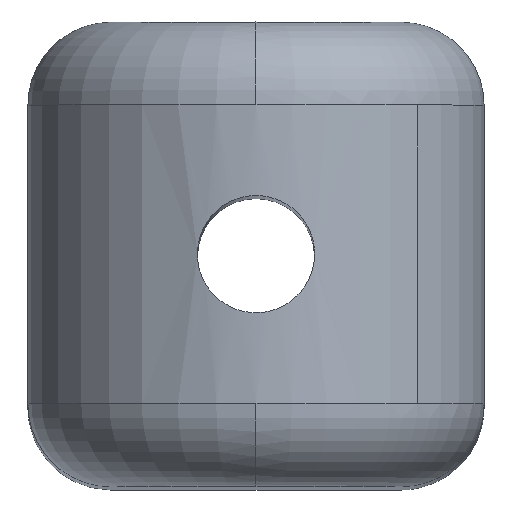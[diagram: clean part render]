
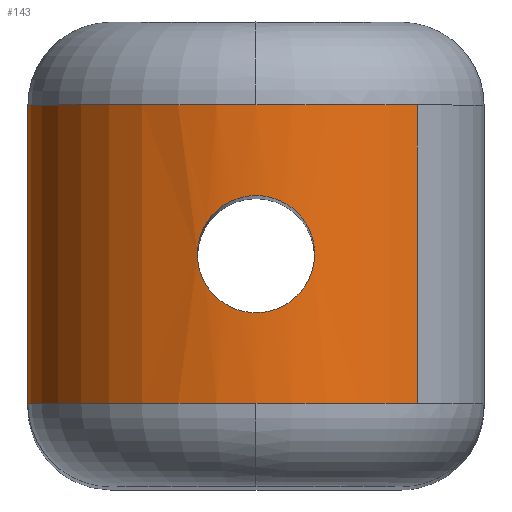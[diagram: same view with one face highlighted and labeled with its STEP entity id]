
A CAD part, top view. The second image highlights one B-rep face of the part: STEP entity #143.
In plain terms, the highlighted cylindrical face has radius 11 mm (diameter 22 mm), a partial arc.
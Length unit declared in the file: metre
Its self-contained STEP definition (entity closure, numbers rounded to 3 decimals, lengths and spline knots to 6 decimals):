
#143=ADVANCED_FACE('0:40',(#271,#272),#273,.T.);
#271=FACE_OUTER_BOUND('',#383,.T.);
#272=FACE_BOUND('',#384,.T.);
#273=CYLINDRICAL_SURFACE('',#385,0.011);
#383=EDGE_LOOP('',(#640,#641,#642,#643,#644,#645));
#384=EDGE_LOOP('',(#646,#647));
#385=AXIS2_PLACEMENT_3D('',#648,#649,#650);
#640=ORIENTED_EDGE('',*,*,#654,.T.);
#641=ORIENTED_EDGE('',*,*,#660,.F.);
#642=ORIENTED_EDGE('',*,*,#751,.F.);
#643=ORIENTED_EDGE('',*,*,#749,.F.);
#644=ORIENTED_EDGE('',*,*,#747,.F.);
#645=ORIENTED_EDGE('',*,*,#669,.F.);
#646=ORIENTED_EDGE('',*,*,#716,.T.);
#647=ORIENTED_EDGE('',*,*,#702,.T.);
#648=CARTESIAN_POINT('',(0.,0.0,0.099));
#649=DIRECTION('',(0.0,-1.0,0.0));
#650=DIRECTION('',(0.707,0.0,0.707));
#654=EDGE_CURVE('',#755,#756,#757,.T.);
#660=EDGE_CURVE('0:184',#764,#756,#767,.T.);
#669=EDGE_CURVE('0:199',#755,#775,#782,.T.);
#702=EDGE_CURVE('0:4471',#834,#831,#835,.T.);
#716=EDGE_CURVE('0:4471',#831,#834,#854,.T.);
#747=EDGE_CURVE('0:199',#775,#873,#890,.T.);
#749=EDGE_CURVE('0:328',#873,#880,#892,.T.);
#751=EDGE_CURVE('0:184',#880,#764,#894,.T.);
#755=VERTEX_POINT('',#898);
#756=VERTEX_POINT('',#899);
#757=LINE('',#900,#901);
#764=VERTEX_POINT('',#909);
#767=CIRCLE('',#912,0.011);
#775=VERTEX_POINT('',#920);
#782=CIRCLE('',#927,0.011);
#831=VERTEX_POINT('',#990);
#834=VERTEX_POINT('',#994);
#835=B_SPLINE_CURVE_WITH_KNOTS('',3,(#995,#996,#997,#998,#999,#1000,#1001,#1002,#1003,#1004,#1005,#1006,#1007,#1008,#1009,#1010,#1011,#1012,#1013,#1014,#1015,#1016,#1017,#1018,#1019,#1020,#1021,#1022,#1023,#1024,#1025,#1026,#1027,#1028),.UNSPECIFIED.,.F.,.F.,(4,3,3,3,3,3,3,3,3,3,3,4),(0.008555,0.009653,0.010546,0.011007,0.0121,0.012752,0.013258,0.014269,0.014853,0.015323,0.016413,0.017109),.UNSPECIFIED.);
#854=B_SPLINE_CURVE_WITH_KNOTS('',3,(#1050,#1051,#1052,#1053,#1054,#1055,#1056,#1057,#1058,#1059,#1060,#1061,#1062,#1063,#1064,#1065,#1066,#1067,#1068,#1069,#1070,#1071,#1072,#1073,#1074,#1075,#1076,#1077,#1078,#1079,#1080,#1081,#1082,#1083),.UNSPECIFIED.,.F.,.F.,(4,3,3,3,3,3,3,3,3,3,3,4),(0.0,0.001098,0.001991,0.002452,0.003546,0.004197,0.004703,0.005714,0.006298,0.006768,0.007859,0.008555),.UNSPECIFIED.);
#873=VERTEX_POINT('',#1105);
#880=VERTEX_POINT('',#1115);
#890=CIRCLE('',#1127,0.011);
#892=LINE('',#1129,#1130);
#894=CIRCLE('',#1132,0.011);
#898=CARTESIAN_POINT('',(0.007778,-0.0072,0.106778));
#899=CARTESIAN_POINT('',(0.007778,0.0072,0.106778));
#900=CARTESIAN_POINT('',(0.007778,0.0,0.106778));
#901=VECTOR('',#1135,1.0);
#909=CARTESIAN_POINT('',(0.,0.0072,0.11));
#912=AXIS2_PLACEMENT_3D('',#1146,#1147,#1148);
#920=CARTESIAN_POINT('',(0.,-0.0072,0.11));
#927=AXIS2_PLACEMENT_3D('',#1170,#1171,#1172);
#990=CARTESIAN_POINT('',(-0.002825,0.0,0.109631));
#994=CARTESIAN_POINT('',(0.002825,0.,0.109631));
#995=CARTESIAN_POINT('',(0.002825,0.,0.109631));
#996=CARTESIAN_POINT('',(0.002825,-0.000366,0.109631));
#997=CARTESIAN_POINT('',(0.002749,-0.000756,0.109652));
#998=CARTESIAN_POINT('',(0.002597,-0.001111,0.109689));
#999=CARTESIAN_POINT('',(0.002474,-0.0014,0.109719));
#1000=CARTESIAN_POINT('',(0.0023,-0.001667,0.109759));
#1001=CARTESIAN_POINT('',(0.002099,-0.00189,0.109798));
#1002=CARTESIAN_POINT('',(0.001996,-0.002006,0.109818));
#1003=CARTESIAN_POINT('',(0.001885,-0.00211,0.109838));
#1004=CARTESIAN_POINT('',(0.001762,-0.002208,0.109858));
#1005=CARTESIAN_POINT('',(0.00147,-0.002441,0.109905));
#1006=CARTESIAN_POINT('',(0.001117,-0.002623,0.109949));
#1007=CARTESIAN_POINT('',(0.000746,-0.002725,0.109975));
#1008=CARTESIAN_POINT('',(0.000526,-0.002785,0.10999));
#1009=CARTESIAN_POINT('',(0.000299,-0.002818,0.109998));
#1010=CARTESIAN_POINT('',(0.00008,-0.002824,0.11));
#1011=CARTESIAN_POINT('',(-0.00009,-0.002829,0.110001));
#1012=CARTESIAN_POINT('',(-0.00026,-0.002818,0.109998));
#1013=CARTESIAN_POINT('',(-0.000433,-0.002792,0.109991));
#1014=CARTESIAN_POINT('',(-0.000779,-0.002738,0.109978));
#1015=CARTESIAN_POINT('',(-0.001125,-0.002615,0.109947));
#1016=CARTESIAN_POINT('',(-0.00143,-0.002436,0.109907));
#1017=CARTESIAN_POINT('',(-0.001606,-0.002333,0.109884));
#1018=CARTESIAN_POINT('',(-0.001769,-0.002211,0.109858));
#1019=CARTESIAN_POINT('',(-0.001913,-0.002079,0.109832));
#1020=CARTESIAN_POINT('',(-0.002029,-0.001972,0.109812));
#1021=CARTESIAN_POINT('',(-0.002134,-0.001858,0.109791));
#1022=CARTESIAN_POINT('',(-0.002233,-0.001731,0.109771));
#1023=CARTESIAN_POINT('',(-0.002462,-0.001435,0.109724));
#1024=CARTESIAN_POINT('',(-0.002638,-0.00108,0.109679));
#1025=CARTESIAN_POINT('',(-0.002734,-0.00071,0.109655));
#1026=CARTESIAN_POINT('',(-0.002796,-0.000474,0.109639));
#1027=CARTESIAN_POINT('',(-0.002825,-0.000232,0.109631));
#1028=CARTESIAN_POINT('',(-0.002825,0.0,0.109631));
#1050=CARTESIAN_POINT('',(-0.002825,0.0,0.109631));
#1051=CARTESIAN_POINT('',(-0.002825,0.000366,0.109631));
#1052=CARTESIAN_POINT('',(-0.002749,0.000756,0.109652));
#1053=CARTESIAN_POINT('',(-0.002597,0.001111,0.109689));
#1054=CARTESIAN_POINT('',(-0.002474,0.0014,0.109719));
#1055=CARTESIAN_POINT('',(-0.0023,0.001667,0.109759));
#1056=CARTESIAN_POINT('',(-0.002099,0.00189,0.109798));
#1057=CARTESIAN_POINT('',(-0.001996,0.002006,0.109818));
#1058=CARTESIAN_POINT('',(-0.001885,0.00211,0.109838));
#1059=CARTESIAN_POINT('',(-0.001762,0.002208,0.109858));
#1060=CARTESIAN_POINT('',(-0.00147,0.002441,0.109905));
#1061=CARTESIAN_POINT('',(-0.001117,0.002623,0.109949));
#1062=CARTESIAN_POINT('',(-0.000746,0.002725,0.109975));
#1063=CARTESIAN_POINT('',(-0.000526,0.002785,0.10999));
#1064=CARTESIAN_POINT('',(-0.000299,0.002818,0.109998));
#1065=CARTESIAN_POINT('',(-0.00008,0.002824,0.11));
#1066=CARTESIAN_POINT('',(0.00009,0.002829,0.110001));
#1067=CARTESIAN_POINT('',(0.00026,0.002818,0.109998));
#1068=CARTESIAN_POINT('',(0.000433,0.002792,0.109991));
#1069=CARTESIAN_POINT('',(0.000779,0.002738,0.109978));
#1070=CARTESIAN_POINT('',(0.001125,0.002615,0.109947));
#1071=CARTESIAN_POINT('',(0.00143,0.002436,0.109907));
#1072=CARTESIAN_POINT('',(0.001606,0.002333,0.109884));
#1073=CARTESIAN_POINT('',(0.001769,0.002211,0.109858));
#1074=CARTESIAN_POINT('',(0.001913,0.002079,0.109832));
#1075=CARTESIAN_POINT('',(0.002029,0.001972,0.109812));
#1076=CARTESIAN_POINT('',(0.002134,0.001858,0.109791));
#1077=CARTESIAN_POINT('',(0.002233,0.001731,0.109771));
#1078=CARTESIAN_POINT('',(0.002462,0.001435,0.109724));
#1079=CARTESIAN_POINT('',(0.002638,0.00108,0.109679));
#1080=CARTESIAN_POINT('',(0.002734,0.00071,0.109655));
#1081=CARTESIAN_POINT('',(0.002796,0.000474,0.109639));
#1082=CARTESIAN_POINT('',(0.002825,0.000232,0.109631));
#1083=CARTESIAN_POINT('',(0.002825,0.,0.109631));
#1105=CARTESIAN_POINT('',(-0.011,-0.0072,0.099));
#1115=CARTESIAN_POINT('',(-0.011,0.0072,0.099));
#1127=AXIS2_PLACEMENT_3D('',#1271,#1272,#1273);
#1129=CARTESIAN_POINT('',(-0.011,-0.007,0.099));
#1130=VECTOR('',#1274,1.0);
#1132=AXIS2_PLACEMENT_3D('',#1275,#1276,#1277);
#1135=DIRECTION('',(-0.0,1.0,0.0));
#1146=CARTESIAN_POINT('',(0.,0.0072,0.099));
#1147=DIRECTION('',(-0.0,1.0,0.0));
#1148=DIRECTION('',(0.,0.0,1.0));
#1170=CARTESIAN_POINT('',(0.,-0.0072,0.099));
#1171=DIRECTION('',(0.0,-1.0,0.0));
#1172=DIRECTION('',(0.,0.0,1.0));
#1271=CARTESIAN_POINT('',(0.,-0.0072,0.099));
#1272=DIRECTION('',(0.0,-1.0,0.0));
#1273=DIRECTION('',(0.,0.0,1.0));
#1274=DIRECTION('',(0.0,1.0,0.0));
#1275=CARTESIAN_POINT('',(0.,0.0072,0.099));
#1276=DIRECTION('',(-0.0,1.0,0.0));
#1277=DIRECTION('',(0.,0.0,1.0));
